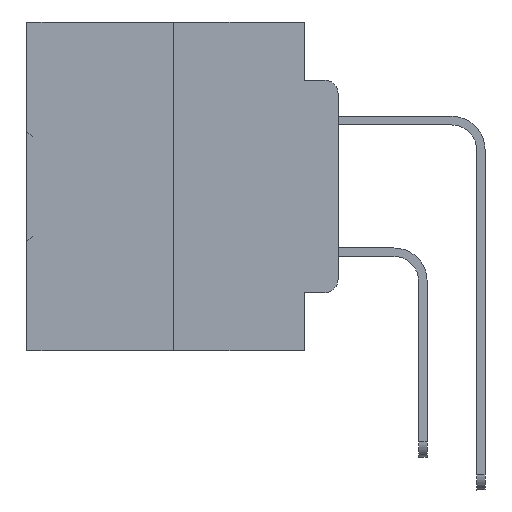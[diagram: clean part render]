
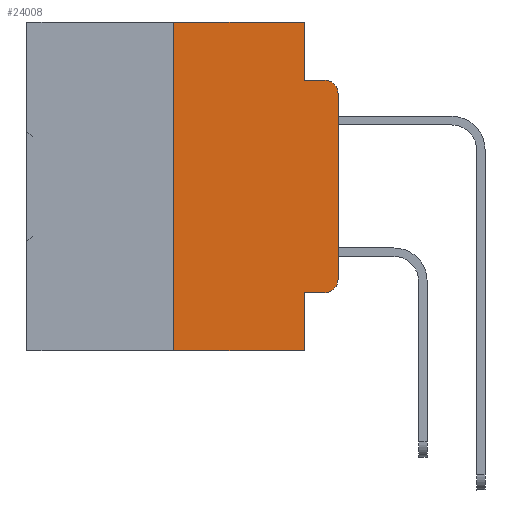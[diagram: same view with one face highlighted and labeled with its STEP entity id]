
A CAD part, left-side view. The second image highlights one B-rep face of the part: STEP entity #24008.
In plain terms, the highlighted planar face has unit normal (-1, 0, 0).
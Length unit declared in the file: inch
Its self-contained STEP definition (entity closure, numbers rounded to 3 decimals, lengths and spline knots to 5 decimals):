
#662 = LINE ( 'NONE', #17107, #23247 ) ;
#1142 = CARTESIAN_POINT ( 'NONE',  ( 0., 0.25, 0. ) ) ;
#1349 = LINE ( 'NONE', #15128, #13353 ) ;
#1572 = CARTESIAN_POINT ( 'NONE',  ( 0., 0.051, -0.5 ) ) ;
#3494 = ORIENTED_EDGE ( 'NONE', *, *, #20276, .F. ) ;
#4584 = VERTEX_POINT ( 'NONE', #5976 ) ;
#4854 = VERTEX_POINT ( 'NONE', #21485 ) ;
#5110 = DIRECTION ( 'NONE',  ( 0., 0., -1. ) ) ;
#5976 = CARTESIAN_POINT ( 'NONE',  ( 0., 0.051, -0.0885 ) ) ;
#7064 = CARTESIAN_POINT ( 'NONE',  ( 0., 0.02, -0.1085 ) ) ;
#7887 = DIRECTION ( 'NONE',  ( 0., 0., -1. ) ) ;
#8379 = EDGE_CURVE ( 'NONE', #22242, #12138, #28613, .T. ) ;
#8512 = CARTESIAN_POINT ( 'NONE',  ( 0., 0.051, -0.4115 ) ) ;
#8669 = VECTOR ( 'NONE', #7887, 39.37008 ) ;
#9522 = EDGE_CURVE ( 'NONE', #24404, #4854, #662, .T. ) ;
#9673 = DIRECTION ( 'NONE',  ( 0., 0., 1. ) ) ;
#9712 = DIRECTION ( 'NONE',  ( 0., 0., -1. ) ) ;
#10215 = VECTOR ( 'NONE', #36556, 39.37008 ) ;
#10358 = AXIS2_PLACEMENT_3D ( 'NONE', #11044, #31309, #5110 ) ;
#10518 = CARTESIAN_POINT ( 'NONE',  ( 0., 0.473, 0. ) ) ;
#11044 = CARTESIAN_POINT ( 'NONE',  ( 0., 0.02, -0.3915 ) ) ;
#11173 = VERTEX_POINT ( 'NONE', #1572 ) ;
#11252 = DIRECTION ( 'NONE',  ( 0., 0., -1. ) ) ;
#11359 = LINE ( 'NONE', #22880, #32033 ) ;
#11884 = ORIENTED_EDGE ( 'NONE', *, *, #8379, .T. ) ;
#12138 = VERTEX_POINT ( 'NONE', #17899 ) ;
#12231 = EDGE_CURVE ( 'NONE', #27927, #17692, #25067, .T. ) ;
#12352 = AXIS2_PLACEMENT_3D ( 'NONE', #7064, #26894, #9712 ) ;
#12357 = VECTOR ( 'NONE', #24192, 39.37008 ) ;
#12962 = ORIENTED_EDGE ( 'NONE', *, *, #17217, .F. ) ;
#13353 = VECTOR ( 'NONE', #9673, 39.37008 ) ;
#14055 = ORIENTED_EDGE ( 'NONE', *, *, #12231, .F. ) ;
#14084 = FACE_OUTER_BOUND ( 'NONE', #34725, .T. ) ;
#14832 = ORIENTED_EDGE ( 'NONE', *, *, #33752, .T. ) ;
#15052 = AXIS2_PLACEMENT_3D ( 'NONE', #10518, #37098, #11252 ) ;
#15128 = CARTESIAN_POINT ( 'NONE',  ( 0., 0., 0. ) ) ;
#16753 = CARTESIAN_POINT ( 'NONE',  ( 0., 0.051, 0. ) ) ;
#17097 = VECTOR ( 'NONE', #19042, 39.37008 ) ;
#17107 = CARTESIAN_POINT ( 'NONE',  ( 0., 0.051, -0.4115 ) ) ;
#17138 = VERTEX_POINT ( 'NONE', #27205 ) ;
#17217 = EDGE_CURVE ( 'NONE', #17138, #27927, #27015, .T. ) ;
#17692 = VERTEX_POINT ( 'NONE', #28599 ) ;
#17709 = VECTOR ( 'NONE', #34761, 39.37008 ) ;
#17899 = CARTESIAN_POINT ( 'NONE',  ( 0., 0.02, -0.0885 ) ) ;
#18795 = ORIENTED_EDGE ( 'NONE', *, *, #21782, .T. ) ;
#19042 = DIRECTION ( 'NONE',  ( 0., 0., -1. ) ) ;
#19497 = ORIENTED_EDGE ( 'NONE', *, *, #23481, .F. ) ;
#19602 = CARTESIAN_POINT ( 'NONE',  ( 0., 0.051, 0. ) ) ;
#20276 = EDGE_CURVE ( 'NONE', #24404, #11173, #27546, .T. ) ;
#21248 = EDGE_CURVE ( 'NONE', #4584, #12138, #11359, .T. ) ;
#21485 = CARTESIAN_POINT ( 'NONE',  ( 0., 0.02, -0.4115 ) ) ;
#21782 = EDGE_CURVE ( 'NONE', #4854, #27856, #26621, .T. ) ;
#22242 = VERTEX_POINT ( 'NONE', #31263 ) ;
#22880 = CARTESIAN_POINT ( 'NONE',  ( 0., 0.051, -0.0885 ) ) ;
#23027 = CARTESIAN_POINT ( 'NONE',  ( 0., 0., -0.3915 ) ) ;
#23161 = DIRECTION ( 'NONE',  ( 0., -1., 0. ) ) ;
#23247 = VECTOR ( 'NONE', #23161, 39.37008 ) ;
#23277 = CARTESIAN_POINT ( 'NONE',  ( 0., 0.473, -0.5 ) ) ;
#23481 = EDGE_CURVE ( 'NONE', #17692, #4584, #28433, .T. ) ;
#24008 = ADVANCED_FACE ( 'NONE', ( #14084 ), #25612, .F. ) ;
#24192 = DIRECTION ( 'NONE',  ( 0., 0., 1. ) ) ;
#24404 = VERTEX_POINT ( 'NONE', #8512 ) ;
#25067 = LINE ( 'NONE', #33367, #10215 ) ;
#25612 = PLANE ( 'NONE',  #15052 ) ;
#26621 = CIRCLE ( 'NONE', #10358, 0.02 ) ;
#26894 = DIRECTION ( 'NONE',  ( -1., 0., 0. ) ) ;
#27015 = LINE ( 'NONE', #1142, #12357 ) ;
#27205 = CARTESIAN_POINT ( 'NONE',  ( 0., 0.25, -0.5 ) ) ;
#27546 = LINE ( 'NONE', #19602, #17097 ) ;
#27856 = VERTEX_POINT ( 'NONE', #23027 ) ;
#27927 = VERTEX_POINT ( 'NONE', #29043 ) ;
#28203 = ORIENTED_EDGE ( 'NONE', *, *, #21248, .F. ) ;
#28433 = LINE ( 'NONE', #16753, #8669 ) ;
#28599 = CARTESIAN_POINT ( 'NONE',  ( 0., 0.051, 0. ) ) ;
#28613 = CIRCLE ( 'NONE', #12352, 0.02 ) ;
#28769 = EDGE_CURVE ( 'NONE', #27856, #22242, #1349, .T. ) ;
#29043 = CARTESIAN_POINT ( 'NONE',  ( 0., 0.25, 0. ) ) ;
#29491 = ORIENTED_EDGE ( 'NONE', *, *, #9522, .T. ) ;
#29529 = ORIENTED_EDGE ( 'NONE', *, *, #28769, .T. ) ;
#31263 = CARTESIAN_POINT ( 'NONE',  ( 0., 0., -0.1085 ) ) ;
#31309 = DIRECTION ( 'NONE',  ( -1., 0., 0. ) ) ;
#32033 = VECTOR ( 'NONE', #36828, 39.37008 ) ;
#33367 = CARTESIAN_POINT ( 'NONE',  ( 0., 0.473, 0. ) ) ;
#33752 = EDGE_CURVE ( 'NONE', #17138, #11173, #36823, .T. ) ;
#34725 = EDGE_LOOP ( 'NONE', ( #29529, #11884, #28203, #19497, #14055, #12962, #14832, #3494, #29491, #18795 ) ) ;
#34761 = DIRECTION ( 'NONE',  ( 0., -1., 0. ) ) ;
#36556 = DIRECTION ( 'NONE',  ( 0., -1., 0. ) ) ;
#36823 = LINE ( 'NONE', #23277, #17709 ) ;
#36828 = DIRECTION ( 'NONE',  ( 0., -1., 0. ) ) ;
#37098 = DIRECTION ( 'NONE',  ( 1., 0., 0. ) ) ;
